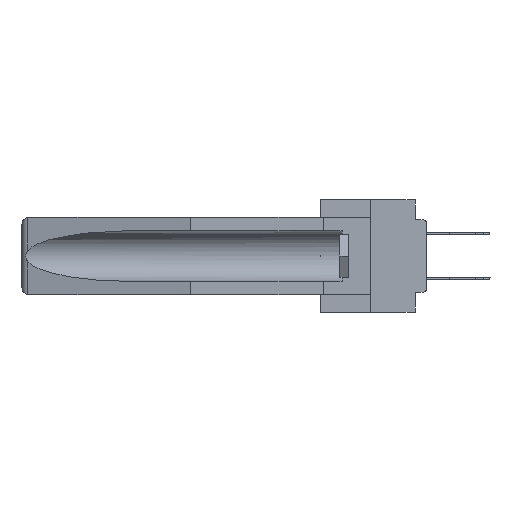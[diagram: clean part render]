
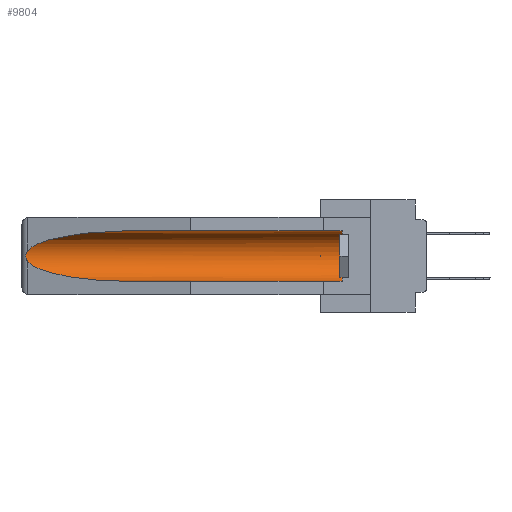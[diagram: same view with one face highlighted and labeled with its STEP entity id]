
A CAD part, left-side view. The second image highlights one B-rep face of the part: STEP entity #9804.
In plain terms, the highlighted cylindrical face has radius 2.857 mm (diameter 5.715 mm), a partial arc.
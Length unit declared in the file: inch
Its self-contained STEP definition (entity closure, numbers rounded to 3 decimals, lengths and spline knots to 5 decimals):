
#701 = CARTESIAN_POINT ( 'NONE',  ( 0.26537, 1.52718, -0.19328 ) ) ;
#1155 = VERTEX_POINT ( 'NONE', #20831 ) ;
#1921 = CARTESIAN_POINT ( 'NONE',  ( 0.26654, 1.53092, -0.15636 ) ) ;
#2167 = VERTEX_POINT ( 'NONE', #11485 ) ;
#2419 = B_SPLINE_CURVE_WITH_KNOTS ( 'NONE', 3,
 ( #11464, #33112, #1921, #22006, #3605, #21621, #25124, #28214, #31039, #27820 ),
 .UNSPECIFIED., .F., .F.,
 ( 4, 2, 2, 2, 4 ),
 ( 0., 0.00029, 0.00058, 0.00087, 0.00117 ),
 .UNSPECIFIED. ) ;
#3524 = EDGE_CURVE ( 'NONE', #20040, #1155, #11651, .T. ) ;
#3600 =( BOUNDED_CURVE ( )  B_SPLINE_CURVE ( 3, ( #11278, #34663, #18727, #20196 ),
 .UNSPECIFIED., .F., .F. ) 
 B_SPLINE_CURVE_WITH_KNOTS ( ( 4, 4 ),
 ( 4.71239, 6.08839 ),
 .UNSPECIFIED. ) 
 CURVE ( )  GEOMETRIC_REPRESENTATION_ITEM ( )  RATIONAL_B_SPLINE_CURVE ( ( 1., 0.848, 0.848, 1. ) ) 
 REPRESENTATION_ITEM ( '' )  );
#3605 = CARTESIAN_POINT ( 'NONE',  ( 0.2675, 1.53308, -0.16763 ) ) ;
#5928 = EDGE_CURVE ( 'NONE', #7227, #1155, #10778, .T. ) ;
#6906 = CARTESIAN_POINT ( 'NONE',  ( 0.155, 1.07973, -0.284 ) ) ;
#7054 = AXIS2_PLACEMENT_3D ( 'NONE', #37393, #22495, #25481 ) ;
#7227 = VERTEX_POINT ( 'NONE', #16986 ) ;
#7742 = EDGE_CURVE ( 'NONE', #2167, #26167, #22796, .T. ) ;
#7929 = CARTESIAN_POINT ( 'NONE',  ( 0.155, 1.07973, -0.059 ) ) ;
#9239 = FACE_OUTER_BOUND ( 'NONE', #13425, .T. ) ;
#9804 = ADVANCED_FACE ( 'NONE', ( #9239 ), #22683, .F. ) ;
#10286 = VERTEX_POINT ( 'NONE', #13625 ) ;
#10778 =( BOUNDED_CURVE ( )  B_SPLINE_CURVE ( 3, ( #701, #28024, #37249, #6906 ),
 .UNSPECIFIED., .F., .F. ) 
 B_SPLINE_CURVE_WITH_KNOTS ( ( 4, 4 ),
 ( 0.1948, 1.5708 ),
 .UNSPECIFIED. ) 
 CURVE ( )  GEOMETRIC_REPRESENTATION_ITEM ( )  RATIONAL_B_SPLINE_CURVE ( ( 1., 0.848, 0.848, 1. ) ) 
 REPRESENTATION_ITEM ( '' )  );
#11273 = EDGE_CURVE ( 'NONE', #20040, #2167, #26444, .T. ) ;
#11278 = CARTESIAN_POINT ( 'NONE',  ( 0.155, 1.07973, -0.059 ) ) ;
#11464 = CARTESIAN_POINT ( 'NONE',  ( 0.26537, 1.52718, -0.14972 ) ) ;
#11485 = CARTESIAN_POINT ( 'NONE',  ( 0.155, 0.126, -0.059 ) ) ;
#11651 = LINE ( 'NONE', #21942, #17410 ) ;
#12362 = CARTESIAN_POINT ( 'NONE',  ( 0.155, 0.126, -0.284 ) ) ;
#13425 = EDGE_LOOP ( 'NONE', ( #35655, #18540, #37286, #30318, #16108, #26946 ) ) ;
#13625 = CARTESIAN_POINT ( 'NONE',  ( 0.26537, 1.52718, -0.14972 ) ) ;
#15657 = EDGE_CURVE ( 'NONE', #10286, #7227, #2419, .T. ) ;
#16108 = ORIENTED_EDGE ( 'NONE', *, *, #11273, .T. ) ;
#16158 = DIRECTION ( 'NONE',  ( 0., 1., 0. ) ) ;
#16986 = CARTESIAN_POINT ( 'NONE',  ( 0.26537, 1.52718, -0.19328 ) ) ;
#17410 = VECTOR ( 'NONE', #25051, 39.37008 ) ;
#18418 = VECTOR ( 'NONE', #16158, 39.37008 ) ;
#18540 = ORIENTED_EDGE ( 'NONE', *, *, #15657, .T. ) ;
#18599 = EDGE_CURVE ( 'NONE', #26167, #10286, #3600, .T. ) ;
#18727 = CARTESIAN_POINT ( 'NONE',  ( 0.25451, 1.48313, -0.09465 ) ) ;
#19654 = CARTESIAN_POINT ( 'NONE',  ( 0.155, -0.30754, -0.059 ) ) ;
#20040 = VERTEX_POINT ( 'NONE', #12362 ) ;
#20196 = CARTESIAN_POINT ( 'NONE',  ( 0.26537, 1.52718, -0.14972 ) ) ;
#20831 = CARTESIAN_POINT ( 'NONE',  ( 0.155, 1.07973, -0.284 ) ) ;
#21621 = CARTESIAN_POINT ( 'NONE',  ( 0.2675, 1.53308, -0.17534 ) ) ;
#21942 = CARTESIAN_POINT ( 'NONE',  ( 0.155, -0.30754, -0.284 ) ) ;
#22006 = CARTESIAN_POINT ( 'NONE',  ( 0.2673, 1.5327, -0.16383 ) ) ;
#22495 = DIRECTION ( 'NONE',  ( 0., 1., 0. ) ) ;
#22683 = CYLINDRICAL_SURFACE ( 'NONE', #7054, 0.1125 ) ;
#22796 = LINE ( 'NONE', #19654, #18418 ) ;
#25051 = DIRECTION ( 'NONE',  ( 0., 1., 0. ) ) ;
#25124 = CARTESIAN_POINT ( 'NONE',  ( 0.2673, 1.53269, -0.17917 ) ) ;
#25481 = DIRECTION ( 'NONE',  ( 0., 0., 1. ) ) ;
#25901 = DIRECTION ( 'NONE',  ( 0., -1., 0. ) ) ;
#26167 = VERTEX_POINT ( 'NONE', #7929 ) ;
#26444 = CIRCLE ( 'NONE', #27961, 0.1125 ) ;
#26946 = ORIENTED_EDGE ( 'NONE', *, *, #7742, .T. ) ;
#27820 = CARTESIAN_POINT ( 'NONE',  ( 0.26537, 1.52718, -0.19328 ) ) ;
#27961 = AXIS2_PLACEMENT_3D ( 'NONE', #34780, #25901, #35446 ) ;
#28024 = CARTESIAN_POINT ( 'NONE',  ( 0.25451, 1.48313, -0.24835 ) ) ;
#28214 = CARTESIAN_POINT ( 'NONE',  ( 0.26655, 1.53094, -0.18657 ) ) ;
#30318 = ORIENTED_EDGE ( 'NONE', *, *, #3524, .F. ) ;
#31039 = CARTESIAN_POINT ( 'NONE',  ( 0.26597, 1.5296, -0.19026 ) ) ;
#33112 = CARTESIAN_POINT ( 'NONE',  ( 0.26597, 1.52961, -0.15275 ) ) ;
#34663 = CARTESIAN_POINT ( 'NONE',  ( 0.21114, 1.30732, -0.059 ) ) ;
#34780 = CARTESIAN_POINT ( 'NONE',  ( 0.155, 0.126, -0.1715 ) ) ;
#35446 = DIRECTION ( 'NONE',  ( 0., 0., 1. ) ) ;
#35655 = ORIENTED_EDGE ( 'NONE', *, *, #18599, .T. ) ;
#37249 = CARTESIAN_POINT ( 'NONE',  ( 0.21114, 1.30732, -0.284 ) ) ;
#37286 = ORIENTED_EDGE ( 'NONE', *, *, #5928, .T. ) ;
#37393 = CARTESIAN_POINT ( 'NONE',  ( 0.155, -0.30754, -0.1715 ) ) ;
